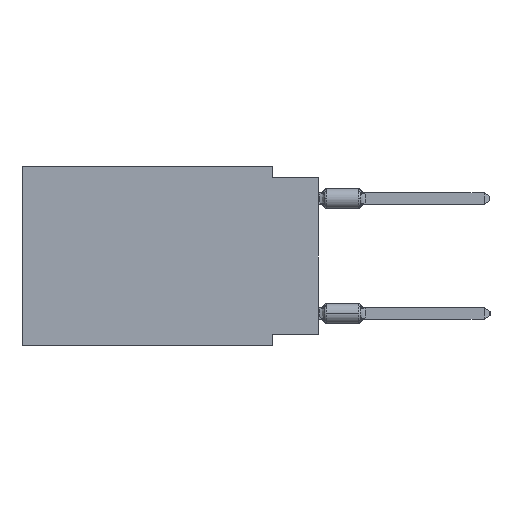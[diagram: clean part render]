
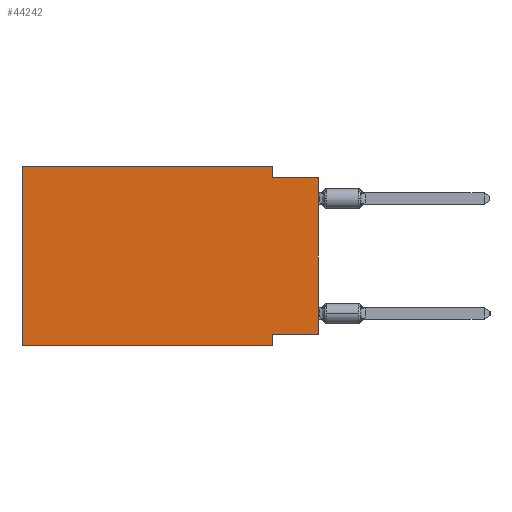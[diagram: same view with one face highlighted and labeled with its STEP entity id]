
A CAD part, left-side view. The second image highlights one B-rep face of the part: STEP entity #44242.
In plain terms, the highlighted planar face has unit normal (-1, 0, 0).
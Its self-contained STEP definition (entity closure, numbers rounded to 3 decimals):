
#235 = LINE ( 'NONE', #26998, #279 ) ;
#279 = VECTOR ( 'NONE', #17157, 1000. ) ;
#983 = CARTESIAN_POINT ( 'NONE',  ( 0., 2.54, -9.906 ) ) ;
#3320 = VECTOR ( 'NONE', #26107, 1000. ) ;
#3843 = VECTOR ( 'NONE', #9981, 1000. ) ;
#4136 = ORIENTED_EDGE ( 'NONE', *, *, #17322, .F. ) ;
#5717 = LINE ( 'NONE', #12101, #25973 ) ;
#6020 = EDGE_CURVE ( 'NONE', #33332, #8640, #20638, .T. ) ;
#7016 = CARTESIAN_POINT ( 'NONE',  ( 0., 0., -0.635 ) ) ;
#7403 = CARTESIAN_POINT ( 'NONE',  ( 0., 2.54, -0.635 ) ) ;
#7643 = FACE_OUTER_BOUND ( 'NONE', #19502, .T. ) ;
#8236 = DIRECTION ( 'NONE',  ( 0., 0., 1. ) ) ;
#8640 = VERTEX_POINT ( 'NONE', #7016 ) ;
#9661 = CARTESIAN_POINT ( 'NONE',  ( 0., 2.54, -9.906 ) ) ;
#9972 = VECTOR ( 'NONE', #38033, 1000. ) ;
#9981 = DIRECTION ( 'NONE',  ( 0., 0., -1. ) ) ;
#10830 = DIRECTION ( 'NONE',  ( 0., 0., -1. ) ) ;
#11326 = VERTEX_POINT ( 'NONE', #30209 ) ;
#11921 = LINE ( 'NONE', #983, #3320 ) ;
#12101 = CARTESIAN_POINT ( 'NONE',  ( 0., 0., -9.271 ) ) ;
#12138 = EDGE_CURVE ( 'NONE', #29458, #8640, #30927, .T. ) ;
#12971 = LINE ( 'NONE', #37006, #3843 ) ;
#13718 = ORIENTED_EDGE ( 'NONE', *, *, #12138, .T. ) ;
#15130 = EDGE_CURVE ( 'NONE', #22299, #18601, #235, .T. ) ;
#16383 = VECTOR ( 'NONE', #8236, 1000. ) ;
#17157 = DIRECTION ( 'NONE',  ( 0., -1., 0. ) ) ;
#17322 = EDGE_CURVE ( 'NONE', #11326, #33681, #11921, .T. ) ;
#17686 = DIRECTION ( 'NONE',  ( 1., 0., 0. ) ) ;
#17869 = ORIENTED_EDGE ( 'NONE', *, *, #36788, .F. ) ;
#18601 = VERTEX_POINT ( 'NONE', #43486 ) ;
#19502 = EDGE_LOOP ( 'NONE', ( #13718, #22917, #28449, #41642, #39419, #33303, #4136, #17869 ) ) ;
#20638 = LINE ( 'NONE', #27294, #9972 ) ;
#21123 = PLANE ( 'NONE',  #34518 ) ;
#22299 = VERTEX_POINT ( 'NONE', #37386 ) ;
#22917 = ORIENTED_EDGE ( 'NONE', *, *, #6020, .F. ) ;
#23366 = LINE ( 'NONE', #26571, #42669 ) ;
#24924 = VECTOR ( 'NONE', #27289, 1000. ) ;
#25101 = VERTEX_POINT ( 'NONE', #33924 ) ;
#25398 = CARTESIAN_POINT ( 'NONE',  ( 0., 16.383, 0. ) ) ;
#25973 = VECTOR ( 'NONE', #26045, 1000. ) ;
#26045 = DIRECTION ( 'NONE',  ( 0., 1., 0. ) ) ;
#26107 = DIRECTION ( 'NONE',  ( 0., 0., -1. ) ) ;
#26571 = CARTESIAN_POINT ( 'NONE',  ( 0., 16.383, -9.906 ) ) ;
#26998 = CARTESIAN_POINT ( 'NONE',  ( 0., 16.383, 0. ) ) ;
#27289 = DIRECTION ( 'NONE',  ( 0., 0., 1. ) ) ;
#27294 = CARTESIAN_POINT ( 'NONE',  ( 0., 0., -0.635 ) ) ;
#28449 = ORIENTED_EDGE ( 'NONE', *, *, #30544, .F. ) ;
#29458 = VERTEX_POINT ( 'NONE', #38327 ) ;
#30004 = DIRECTION ( 'NONE',  ( 0., -1., 0. ) ) ;
#30209 = CARTESIAN_POINT ( 'NONE',  ( 0., 2.54, -9.271 ) ) ;
#30544 = EDGE_CURVE ( 'NONE', #18601, #33332, #12971, .T. ) ;
#30927 = LINE ( 'NONE', #33487, #24924 ) ;
#32653 = EDGE_CURVE ( 'NONE', #25101, #33681, #23366, .T. ) ;
#32902 = EDGE_CURVE ( 'NONE', #25101, #22299, #39362, .T. ) ;
#33303 = ORIENTED_EDGE ( 'NONE', *, *, #32653, .T. ) ;
#33332 = VERTEX_POINT ( 'NONE', #7403 ) ;
#33487 = CARTESIAN_POINT ( 'NONE',  ( 0., 0., 0. ) ) ;
#33681 = VERTEX_POINT ( 'NONE', #9661 ) ;
#33924 = CARTESIAN_POINT ( 'NONE',  ( 0., 16.383, -9.906 ) ) ;
#34518 = AXIS2_PLACEMENT_3D ( 'NONE', #35071, #17686, #10830 ) ;
#35071 = CARTESIAN_POINT ( 'NONE',  ( 0., 16.383, 0. ) ) ;
#36788 = EDGE_CURVE ( 'NONE', #29458, #11326, #5717, .T. ) ;
#37006 = CARTESIAN_POINT ( 'NONE',  ( 0., 2.54, 0. ) ) ;
#37386 = CARTESIAN_POINT ( 'NONE',  ( 0., 16.383, 0. ) ) ;
#38033 = DIRECTION ( 'NONE',  ( 0., -1., 0. ) ) ;
#38327 = CARTESIAN_POINT ( 'NONE',  ( 0., 0., -9.271 ) ) ;
#39362 = LINE ( 'NONE', #25398, #16383 ) ;
#39419 = ORIENTED_EDGE ( 'NONE', *, *, #32902, .F. ) ;
#41642 = ORIENTED_EDGE ( 'NONE', *, *, #15130, .F. ) ;
#42669 = VECTOR ( 'NONE', #30004, 1000. ) ;
#43486 = CARTESIAN_POINT ( 'NONE',  ( 0., 2.54, 0. ) ) ;
#44242 = ADVANCED_FACE ( 'NONE', ( #7643 ), #21123, .F. ) ;
